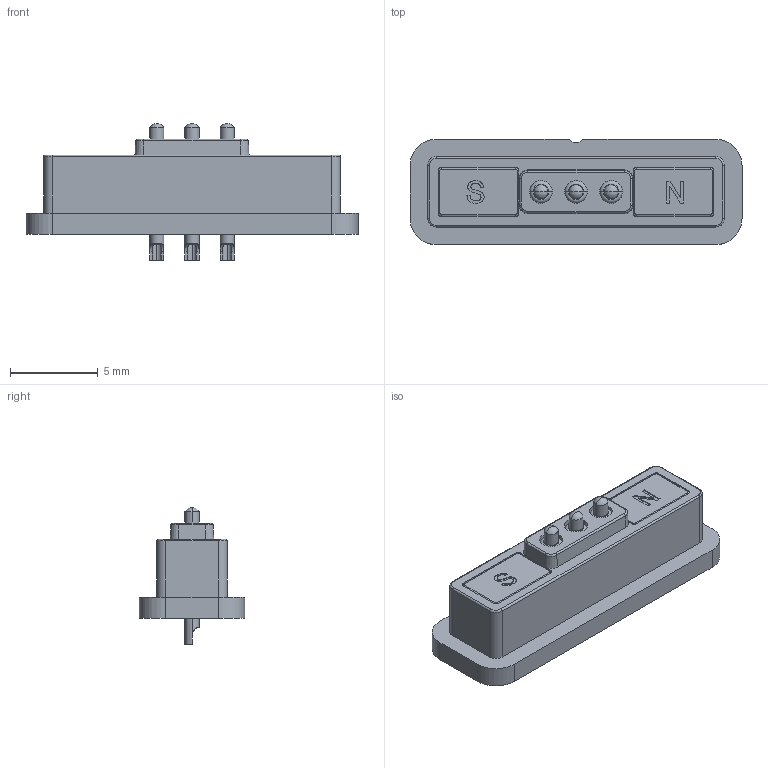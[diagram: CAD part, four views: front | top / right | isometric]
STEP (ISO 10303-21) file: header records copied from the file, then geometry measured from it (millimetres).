
FILE_DESCRIPTION (( 'STEP AP203' ), '1' );
FILE_NAME ('685-F0321451110.STEP', '2023-02-14T05:57:48', ( 'Magnum' ), ( '' ), 'SwSTEP 2.0', 'SolidWorks 2020', '' );
FILE_SCHEMA (( 'CONFIG_CONTROL_DESIGN' ));
Length unit declared in the file: millimetre
Products named in the file (1): 685-F0321451110
Bounding box: 18.9 x 6 x 7.8 mm (x, y, z)
Volume: 340.4 mm3; surface area: 617.8 mm2
Topology: 4 solids, 9 shells, 258 faces, 601 edges, 367 vertices
Faces by surface type: cylinder 102, plane 90, torus 30, cone 16, bspline 14, sphere 6
Entity records: 8453 total; most frequent: CARTESIAN_POINT 2440, DIRECTION 1290, ORIENTED_EDGE 1190, EDGE_CURVE 595, AXIS2_PLACEMENT_3D 487, VERTEX_POINT 367, LINE 316, VECTOR 316
